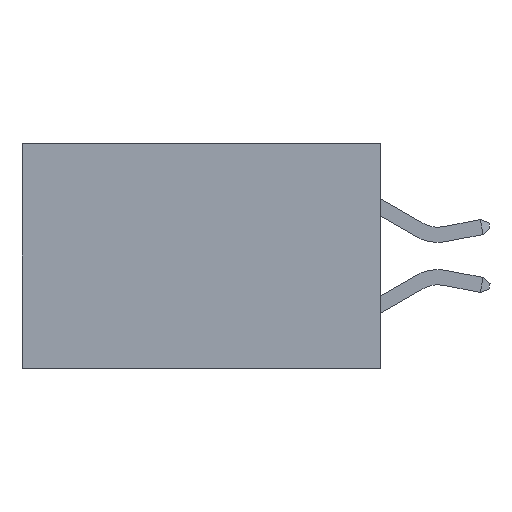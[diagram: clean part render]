
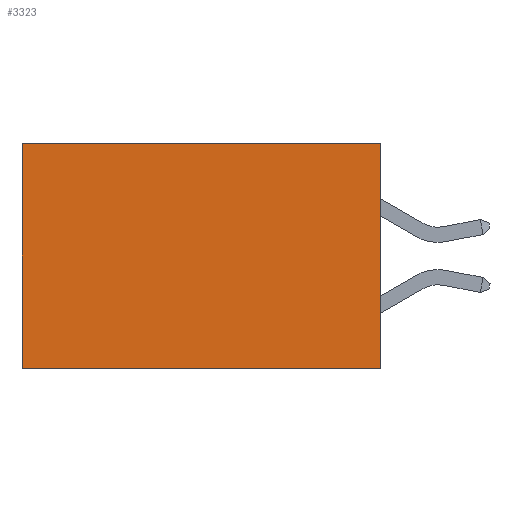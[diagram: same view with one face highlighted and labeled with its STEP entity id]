
A CAD part, left-side view. The second image highlights one B-rep face of the part: STEP entity #3323.
In plain terms, the highlighted planar face has unit normal (-1, 0, 0).
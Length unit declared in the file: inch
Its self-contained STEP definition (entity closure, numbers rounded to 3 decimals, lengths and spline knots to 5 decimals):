
#187 = FACE_OUTER_BOUND ( 'NONE', #2394, .T. ) ;
#650 = EDGE_CURVE ( 'NONE', #6965, #6848, #7875, .T. ) ;
#664 = CARTESIAN_POINT ( 'NONE',  ( 0.277, 0., -0.37 ) ) ;
#986 = CARTESIAN_POINT ( 'NONE',  ( 0.277, 0., 0. ) ) ;
#1030 = ORIENTED_EDGE ( 'NONE', *, *, #5079, .T. ) ;
#1105 = CARTESIAN_POINT ( 'NONE',  ( 0.277, 0., -0.37 ) ) ;
#1281 = AXIS2_PLACEMENT_3D ( 'NONE', #4867, #4652, #4624 ) ;
#1380 = ORIENTED_EDGE ( 'NONE', *, *, #650, .F. ) ;
#1442 = CARTESIAN_POINT ( 'NONE',  ( 0.277, 0.59, -0.37 ) ) ;
#2109 = CARTESIAN_POINT ( 'NONE',  ( 0.277, 0.59, 0. ) ) ;
#2394 = EDGE_LOOP ( 'NONE', ( #1030, #1380, #7709, #7015 ) ) ;
#2882 = VECTOR ( 'NONE', #5614, 39.37008 ) ;
#3224 = VECTOR ( 'NONE', #4070, 39.37008 ) ;
#3323 = ADVANCED_FACE ( 'NONE', ( #187 ), #4974, .F. ) ;
#3990 = VERTEX_POINT ( 'NONE', #2109 ) ;
#4070 = DIRECTION ( 'NONE',  ( 0., 0., -1. ) ) ;
#4252 = CARTESIAN_POINT ( 'NONE',  ( 0.277, 0.59, -0.37 ) ) ;
#4624 = DIRECTION ( 'NONE',  ( 0., 0., -1. ) ) ;
#4652 = DIRECTION ( 'NONE',  ( 1., 0., 0. ) ) ;
#4867 = CARTESIAN_POINT ( 'NONE',  ( 0.277, 0., -0.37 ) ) ;
#4974 = PLANE ( 'NONE',  #1281 ) ;
#5079 = EDGE_CURVE ( 'NONE', #3990, #6848, #8349, .T. ) ;
#5116 = DIRECTION ( 'NONE',  ( 0., 1., 0. ) ) ;
#5517 = VECTOR ( 'NONE', #6122, 39.37008 ) ;
#5614 = DIRECTION ( 'NONE',  ( 0., 0., -1. ) ) ;
#6122 = DIRECTION ( 'NONE',  ( 0., 1., 0. ) ) ;
#6150 = VECTOR ( 'NONE', #5116, 39.37008 ) ;
#6398 = EDGE_CURVE ( 'NONE', #7505, #3990, #7039, .T. ) ;
#6848 = VERTEX_POINT ( 'NONE', #1442 ) ;
#6965 = VERTEX_POINT ( 'NONE', #7950 ) ;
#7015 = ORIENTED_EDGE ( 'NONE', *, *, #6398, .T. ) ;
#7039 = LINE ( 'NONE', #986, #5517 ) ;
#7231 = EDGE_CURVE ( 'NONE', #7505, #6965, #7624, .T. ) ;
#7505 = VERTEX_POINT ( 'NONE', #7585 ) ;
#7585 = CARTESIAN_POINT ( 'NONE',  ( 0.277, 0., 0. ) ) ;
#7624 = LINE ( 'NONE', #1105, #2882 ) ;
#7709 = ORIENTED_EDGE ( 'NONE', *, *, #7231, .F. ) ;
#7875 = LINE ( 'NONE', #664, #6150 ) ;
#7950 = CARTESIAN_POINT ( 'NONE',  ( 0.277, 0., -0.37 ) ) ;
#8349 = LINE ( 'NONE', #4252, #3224 ) ;
